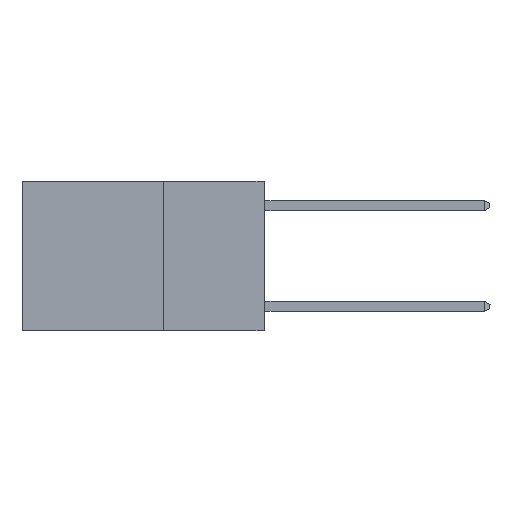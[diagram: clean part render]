
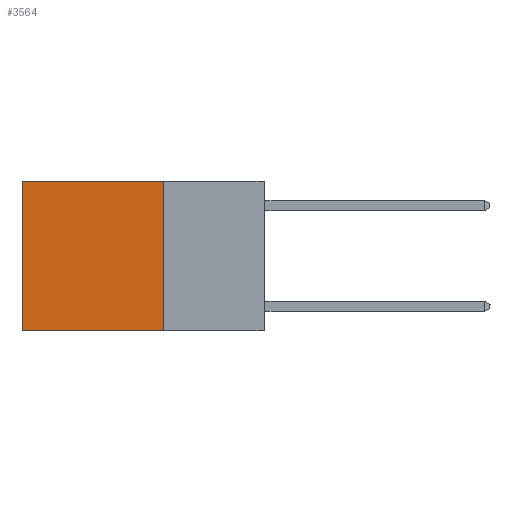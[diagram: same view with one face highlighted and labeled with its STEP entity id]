
A CAD part, left-side view. The second image highlights one B-rep face of the part: STEP entity #3564.
In plain terms, the highlighted planar face has unit normal (-1, 0, 0).
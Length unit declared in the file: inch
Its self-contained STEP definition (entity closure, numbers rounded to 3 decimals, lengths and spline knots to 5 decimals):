
#113 = EDGE_CURVE ( 'NONE', #301, #2438, #6285, .T. ) ;
#301 = VERTEX_POINT ( 'NONE', #3979 ) ;
#396 = CARTESIAN_POINT ( 'NONE',  ( 0.2625, 0.25, -0.37 ) ) ;
#559 = PLANE ( 'NONE',  #8862 ) ;
#788 = DIRECTION ( 'NONE',  ( 0., 1., 0. ) ) ;
#1312 = VECTOR ( 'NONE', #4905, 39.37008 ) ;
#1545 = CARTESIAN_POINT ( 'NONE',  ( 0.2625, 0.25, 0. ) ) ;
#1641 = VECTOR ( 'NONE', #10359, 39.37008 ) ;
#1842 = LINE ( 'NONE', #4652, #8330 ) ;
#1867 = FACE_OUTER_BOUND ( 'NONE', #5504, .T. ) ;
#2426 = VERTEX_POINT ( 'NONE', #10043 ) ;
#2438 = VERTEX_POINT ( 'NONE', #396 ) ;
#3431 = DIRECTION ( 'NONE',  ( 0., 0., -1. ) ) ;
#3564 = ADVANCED_FACE ( 'NONE', ( #1867 ), #559, .F. ) ;
#3624 = LINE ( 'NONE', #4872, #1312 ) ;
#3979 = CARTESIAN_POINT ( 'NONE',  ( 0.2625, 0.25, 0. ) ) ;
#4096 = EDGE_CURVE ( 'NONE', #2438, #7943, #1842, .T. ) ;
#4421 = EDGE_CURVE ( 'NONE', #2426, #7943, #7547, .T. ) ;
#4491 = DIRECTION ( 'NONE',  ( 0., 0., -1. ) ) ;
#4652 = CARTESIAN_POINT ( 'NONE',  ( 0.2625, 0.25, -0.37 ) ) ;
#4697 = ORIENTED_EDGE ( 'NONE', *, *, #113, .F. ) ;
#4872 = CARTESIAN_POINT ( 'NONE',  ( 0.2625, 0.25, 0. ) ) ;
#4905 = DIRECTION ( 'NONE',  ( 0., 1., 0. ) ) ;
#5291 = CARTESIAN_POINT ( 'NONE',  ( 0.2625, 0.6, 0. ) ) ;
#5504 = EDGE_LOOP ( 'NONE', ( #7670, #8327, #4697, #10646 ) ) ;
#5638 = VECTOR ( 'NONE', #3431, 39.37008 ) ;
#6062 = CARTESIAN_POINT ( 'NONE',  ( 0.2625, 0.6, -0.37 ) ) ;
#6285 = LINE ( 'NONE', #1545, #1641 ) ;
#7547 = LINE ( 'NONE', #5291, #5638 ) ;
#7670 = ORIENTED_EDGE ( 'NONE', *, *, #4421, .T. ) ;
#7700 = EDGE_CURVE ( 'NONE', #301, #2426, #3624, .T. ) ;
#7943 = VERTEX_POINT ( 'NONE', #6062 ) ;
#8327 = ORIENTED_EDGE ( 'NONE', *, *, #4096, .F. ) ;
#8330 = VECTOR ( 'NONE', #788, 39.37008 ) ;
#8573 = CARTESIAN_POINT ( 'NONE',  ( 0.2625, 0.25, 0. ) ) ;
#8862 = AXIS2_PLACEMENT_3D ( 'NONE', #8573, #9430, #4491 ) ;
#9430 = DIRECTION ( 'NONE',  ( 1., 0., 0. ) ) ;
#10043 = CARTESIAN_POINT ( 'NONE',  ( 0.2625, 0.6, 0. ) ) ;
#10359 = DIRECTION ( 'NONE',  ( 0., 0., -1. ) ) ;
#10646 = ORIENTED_EDGE ( 'NONE', *, *, #7700, .T. ) ;
